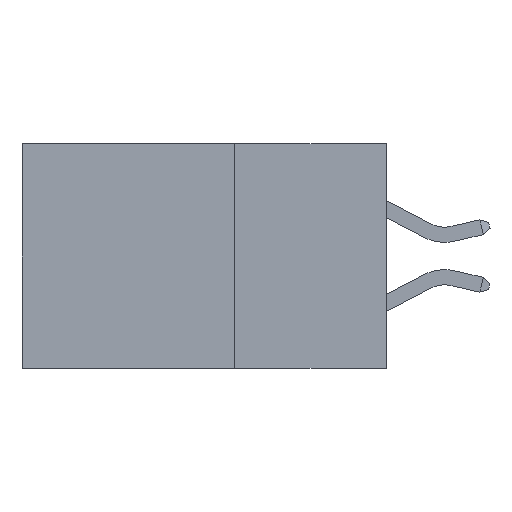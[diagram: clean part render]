
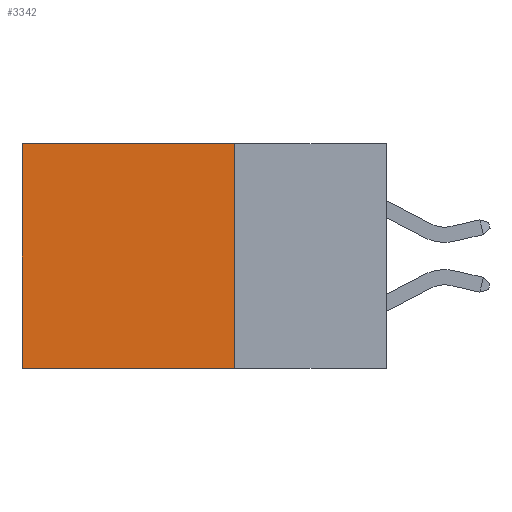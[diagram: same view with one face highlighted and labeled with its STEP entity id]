
A CAD part, left-side view. The second image highlights one B-rep face of the part: STEP entity #3342.
In plain terms, the highlighted planar face has unit normal (-1, 0, 0).
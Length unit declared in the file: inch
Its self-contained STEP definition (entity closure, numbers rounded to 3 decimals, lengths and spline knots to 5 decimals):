
#149 = AXIS2_PLACEMENT_3D ( 'NONE', #15343, #2184, #15446 ) ;
#448 = DIRECTION ( 'NONE',  ( 0., 1., 0. ) ) ;
#666 = CARTESIAN_POINT ( 'NONE',  ( 0.2615, 0.25, 0. ) ) ;
#1454 = ORIENTED_EDGE ( 'NONE', *, *, #12976, .T. ) ;
#1850 = CARTESIAN_POINT ( 'NONE',  ( 0.2615, 0.25, -0.37 ) ) ;
#2081 = FACE_OUTER_BOUND ( 'NONE', #6654, .T. ) ;
#2184 = DIRECTION ( 'NONE',  ( 1., 0., 0. ) ) ;
#2279 = CARTESIAN_POINT ( 'NONE',  ( 0.2615, 0.25, -0.37 ) ) ;
#3136 = LINE ( 'NONE', #5840, #7123 ) ;
#3342 = ADVANCED_FACE ( 'NONE', ( #2081 ), #12739, .F. ) ;
#4213 = EDGE_CURVE ( 'NONE', #7930, #5114, #10437, .T. ) ;
#5039 = LINE ( 'NONE', #17035, #5752 ) ;
#5114 = VERTEX_POINT ( 'NONE', #12778 ) ;
#5123 = DIRECTION ( 'NONE',  ( 0., 1., 0. ) ) ;
#5248 = VERTEX_POINT ( 'NONE', #666 ) ;
#5637 = ORIENTED_EDGE ( 'NONE', *, *, #12416, .F. ) ;
#5752 = VECTOR ( 'NONE', #5123, 39.37008 ) ;
#5777 = VECTOR ( 'NONE', #15728, 39.37008 ) ;
#5840 = CARTESIAN_POINT ( 'NONE',  ( 0.2615, 0.25, -0.37 ) ) ;
#6654 = EDGE_LOOP ( 'NONE', ( #11901, #16346, #5637, #1454 ) ) ;
#7123 = VECTOR ( 'NONE', #9479, 39.37008 ) ;
#7930 = VERTEX_POINT ( 'NONE', #8753 ) ;
#8651 = VERTEX_POINT ( 'NONE', #2279 ) ;
#8753 = CARTESIAN_POINT ( 'NONE',  ( 0.2615, 0.6, 0. ) ) ;
#9479 = DIRECTION ( 'NONE',  ( 0., 0., -1. ) ) ;
#10437 = LINE ( 'NONE', #13117, #5777 ) ;
#11311 = EDGE_CURVE ( 'NONE', #8651, #5114, #16153, .T. ) ;
#11901 = ORIENTED_EDGE ( 'NONE', *, *, #4213, .T. ) ;
#12416 = EDGE_CURVE ( 'NONE', #5248, #8651, #3136, .T. ) ;
#12739 = PLANE ( 'NONE',  #149 ) ;
#12778 = CARTESIAN_POINT ( 'NONE',  ( 0.2615, 0.6, -0.37 ) ) ;
#12976 = EDGE_CURVE ( 'NONE', #5248, #7930, #5039, .T. ) ;
#13117 = CARTESIAN_POINT ( 'NONE',  ( 0.2615, 0.6, -0.37 ) ) ;
#15343 = CARTESIAN_POINT ( 'NONE',  ( 0.2615, 0.25, -0.37 ) ) ;
#15446 = DIRECTION ( 'NONE',  ( 0., 0., -1. ) ) ;
#15728 = DIRECTION ( 'NONE',  ( 0., 0., -1. ) ) ;
#16153 = LINE ( 'NONE', #1850, #16518 ) ;
#16346 = ORIENTED_EDGE ( 'NONE', *, *, #11311, .F. ) ;
#16518 = VECTOR ( 'NONE', #448, 39.37008 ) ;
#17035 = CARTESIAN_POINT ( 'NONE',  ( 0.2615, 0.25, 0. ) ) ;
